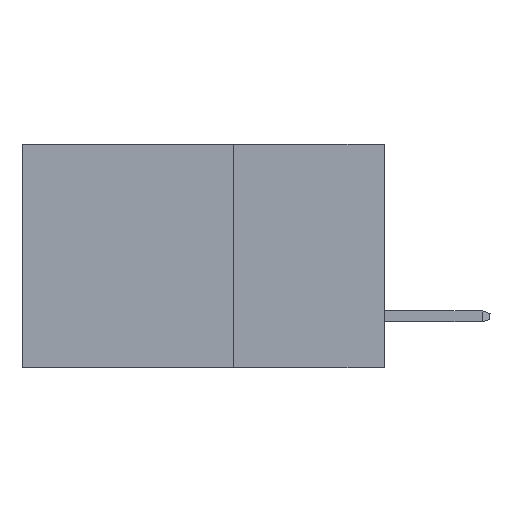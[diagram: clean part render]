
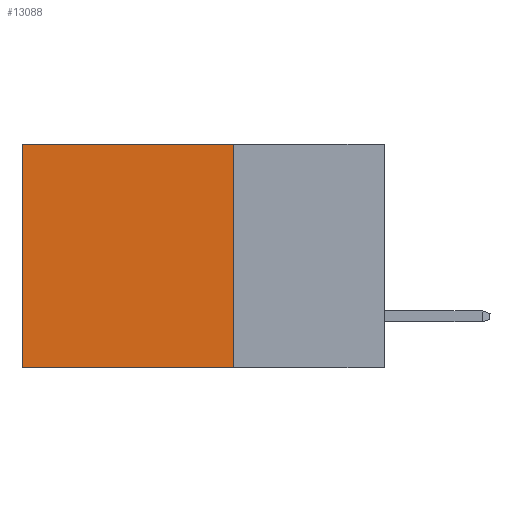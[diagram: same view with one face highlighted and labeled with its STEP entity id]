
A CAD part, left-side view. The second image highlights one B-rep face of the part: STEP entity #13088.
In plain terms, the highlighted planar face has unit normal (-1, 0, 0).
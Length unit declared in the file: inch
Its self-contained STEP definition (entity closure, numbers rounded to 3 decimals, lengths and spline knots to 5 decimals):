
#1559 = EDGE_CURVE ( 'NONE', #2761, #23356, #27733, .T. ) ;
#2298 = CARTESIAN_POINT ( 'NONE',  ( 0.298, 0.6, 0. ) ) ;
#2362 = CARTESIAN_POINT ( 'NONE',  ( 0.298, 0.25, 0. ) ) ;
#2761 = VERTEX_POINT ( 'NONE', #19309 ) ;
#3082 = EDGE_CURVE ( 'NONE', #2761, #8416, #19529, .T. ) ;
#3378 = ORIENTED_EDGE ( 'NONE', *, *, #26315, .F. ) ;
#4282 = LINE ( 'NONE', #13700, #29013 ) ;
#4663 = DIRECTION ( 'NONE',  ( 0., 0., -1. ) ) ;
#5283 = CARTESIAN_POINT ( 'NONE',  ( 0.298, 0.6, 0. ) ) ;
#5878 = DIRECTION ( 'NONE',  ( 0., 0., -1. ) ) ;
#6256 = VECTOR ( 'NONE', #4663, 39.37008 ) ;
#8416 = VERTEX_POINT ( 'NONE', #2298 ) ;
#8698 = DIRECTION ( 'NONE',  ( 0., 1., 0. ) ) ;
#10266 = VECTOR ( 'NONE', #24857, 39.37008 ) ;
#11057 = VERTEX_POINT ( 'NONE', #28920 ) ;
#11323 = CARTESIAN_POINT ( 'NONE',  ( 0.298, 0.25, -0.37 ) ) ;
#13088 = ADVANCED_FACE ( 'NONE', ( #15605 ), #26559, .F. ) ;
#13700 = CARTESIAN_POINT ( 'NONE',  ( 0.298, 0.25, -0.37 ) ) ;
#14952 = VECTOR ( 'NONE', #19826, 39.37008 ) ;
#15413 = CARTESIAN_POINT ( 'NONE',  ( 0.298, 0.25, 0. ) ) ;
#15605 = FACE_OUTER_BOUND ( 'NONE', #26036, .T. ) ;
#19309 = CARTESIAN_POINT ( 'NONE',  ( 0.298, 0.25, 0. ) ) ;
#19529 = LINE ( 'NONE', #15413, #14952 ) ;
#19826 = DIRECTION ( 'NONE',  ( 0., 1., 0. ) ) ;
#21084 = LINE ( 'NONE', #5283, #6256 ) ;
#23356 = VERTEX_POINT ( 'NONE', #11323 ) ;
#24857 = DIRECTION ( 'NONE',  ( 0., 0., -1. ) ) ;
#25923 = ORIENTED_EDGE ( 'NONE', *, *, #3082, .T. ) ;
#26036 = EDGE_LOOP ( 'NONE', ( #29084, #3378, #27957, #25923 ) ) ;
#26315 = EDGE_CURVE ( 'NONE', #23356, #11057, #4282, .T. ) ;
#26419 = AXIS2_PLACEMENT_3D ( 'NONE', #26708, #29431, #5878 ) ;
#26559 = PLANE ( 'NONE',  #26419 ) ;
#26708 = CARTESIAN_POINT ( 'NONE',  ( 0.298, 0.25, 0. ) ) ;
#27733 = LINE ( 'NONE', #2362, #10266 ) ;
#27957 = ORIENTED_EDGE ( 'NONE', *, *, #1559, .F. ) ;
#28920 = CARTESIAN_POINT ( 'NONE',  ( 0.298, 0.6, -0.37 ) ) ;
#29013 = VECTOR ( 'NONE', #8698, 39.37008 ) ;
#29084 = ORIENTED_EDGE ( 'NONE', *, *, #29156, .T. ) ;
#29156 = EDGE_CURVE ( 'NONE', #8416, #11057, #21084, .T. ) ;
#29431 = DIRECTION ( 'NONE',  ( 1., 0., 0. ) ) ;
